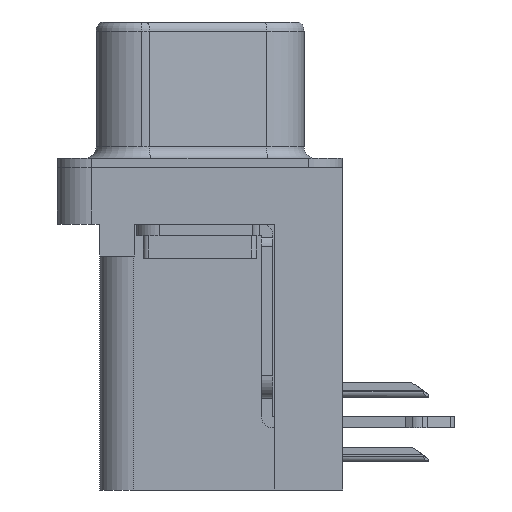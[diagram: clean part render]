
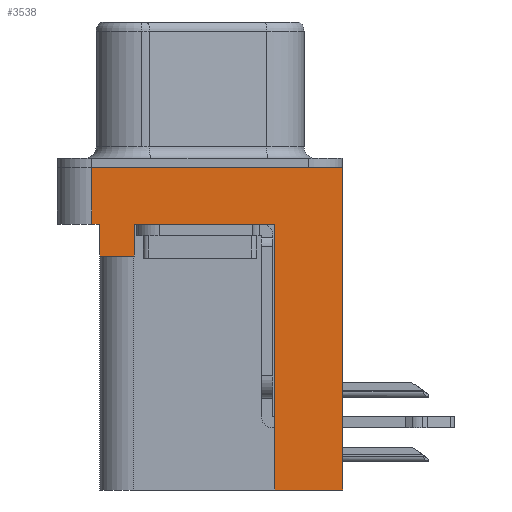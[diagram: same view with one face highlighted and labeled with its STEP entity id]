
A CAD part, left-side view. The second image highlights one B-rep face of the part: STEP entity #3538.
In plain terms, the highlighted planar face has unit normal (-1, 0, 0).
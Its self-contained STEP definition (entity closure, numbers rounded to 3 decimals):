
#238 = LINE ( 'NONE', #12211, #2899 ) ;
#440 = EDGE_CURVE ( 'NONE', #10118, #19211, #15057, .T. ) ;
#524 = CARTESIAN_POINT ( 'NONE',  ( -2.91, 4.775, -2.5 ) ) ;
#968 = DIRECTION ( 'NONE',  ( 0., -1., 0. ) ) ;
#1607 = CARTESIAN_POINT ( 'NONE',  ( -2.91, -3.295, -14.2 ) ) ;
#1790 = DIRECTION ( 'NONE',  ( 0., -1., 0. ) ) ;
#1872 = CARTESIAN_POINT ( 'NONE',  ( -2.91, -6.275, -14.2 ) ) ;
#1928 = LINE ( 'NONE', #10329, #10955 ) ;
#2899 = VECTOR ( 'NONE', #23032, 1000. ) ;
#2955 = ORIENTED_EDGE ( 'NONE', *, *, #18071, .F. ) ;
#3236 = FACE_OUTER_BOUND ( 'NONE', #4705, .T. ) ;
#3308 = VERTEX_POINT ( 'NONE', #25746 ) ;
#3538 = ADVANCED_FACE ( 'NONE', ( #3236 ), #11622, .T. ) ;
#3618 = CARTESIAN_POINT ( 'NONE',  ( -2.91, -3.295, -2.5 ) ) ;
#3626 = ORIENTED_EDGE ( 'NONE', *, *, #4228, .F. ) ;
#4175 = CARTESIAN_POINT ( 'NONE',  ( -2.91, 4.775, 0. ) ) ;
#4181 = ORIENTED_EDGE ( 'NONE', *, *, #12419, .T. ) ;
#4228 = EDGE_CURVE ( 'NONE', #21838, #14316, #9188, .T. ) ;
#4274 = EDGE_CURVE ( 'NONE', #10118, #15035, #8918, .T. ) ;
#4481 = VERTEX_POINT ( 'NONE', #1872 ) ;
#4495 = DIRECTION ( 'NONE',  ( 0., 0., 1. ) ) ;
#4705 = EDGE_LOOP ( 'NONE', ( #24730, #3626, #4181, #11059, #13642, #17425, #17779, #13672, #2955, #18287 ) ) ;
#5242 = VERTEX_POINT ( 'NONE', #1607 ) ;
#6165 = CARTESIAN_POINT ( 'NONE',  ( -2.91, -3.295, -14.2 ) ) ;
#6808 = LINE ( 'NONE', #7444, #15764 ) ;
#7237 = CARTESIAN_POINT ( 'NONE',  ( -2.91, 2.895, -2.5 ) ) ;
#7444 = CARTESIAN_POINT ( 'NONE',  ( -2.91, -6.275, -2.5 ) ) ;
#7488 = DIRECTION ( 'NONE',  ( 0., 0., 1. ) ) ;
#7683 = CARTESIAN_POINT ( 'NONE',  ( -2.91, 4.425, -3.9 ) ) ;
#7937 = EDGE_CURVE ( 'NONE', #5242, #17884, #26872, .T. ) ;
#8073 = DIRECTION ( 'NONE',  ( 0., 0., 1. ) ) ;
#8788 = VECTOR ( 'NONE', #19733, 1000. ) ;
#8872 = DIRECTION ( 'NONE',  ( 0., 0., 1. ) ) ;
#8918 = LINE ( 'NONE', #9320, #22481 ) ;
#9188 = LINE ( 'NONE', #524, #23735 ) ;
#9320 = CARTESIAN_POINT ( 'NONE',  ( -2.91, 4.425, -3.9 ) ) ;
#9418 = VECTOR ( 'NONE', #8073, 1000. ) ;
#10118 = VERTEX_POINT ( 'NONE', #10453 ) ;
#10329 = CARTESIAN_POINT ( 'NONE',  ( -2.91, -6.275, 0. ) ) ;
#10453 = CARTESIAN_POINT ( 'NONE',  ( -2.91, 2.895, -3.9 ) ) ;
#10955 = VECTOR ( 'NONE', #1790, 1000. ) ;
#11059 = ORIENTED_EDGE ( 'NONE', *, *, #20210, .F. ) ;
#11490 = CARTESIAN_POINT ( 'NONE',  ( -2.91, 4.775, -2.5 ) ) ;
#11622 = PLANE ( 'NONE',  #13136 ) ;
#11770 = EDGE_CURVE ( 'NONE', #4481, #17415, #6808, .T. ) ;
#11969 = EDGE_CURVE ( 'NONE', #14316, #17415, #1928, .T. ) ;
#12211 = CARTESIAN_POINT ( 'NONE',  ( -2.91, 4.425, -3.9 ) ) ;
#12419 = EDGE_CURVE ( 'NONE', #21838, #3308, #17669, .T. ) ;
#13136 = AXIS2_PLACEMENT_3D ( 'NONE', #26284, #17925, #7488 ) ;
#13312 = DIRECTION ( 'NONE',  ( 0., 1., 0. ) ) ;
#13642 = ORIENTED_EDGE ( 'NONE', *, *, #4274, .F. ) ;
#13672 = ORIENTED_EDGE ( 'NONE', *, *, #7937, .F. ) ;
#13702 = CARTESIAN_POINT ( 'NONE',  ( -2.91, -6.275, -2.5 ) ) ;
#14316 = VERTEX_POINT ( 'NONE', #4175 ) ;
#15035 = VERTEX_POINT ( 'NONE', #7683 ) ;
#15057 = LINE ( 'NONE', #26738, #26340 ) ;
#15143 = CARTESIAN_POINT ( 'NONE',  ( -2.91, -3.295, -14.2 ) ) ;
#15764 = VECTOR ( 'NONE', #4495, 1000. ) ;
#16016 = CARTESIAN_POINT ( 'NONE',  ( -2.91, -6.275, 0. ) ) ;
#17415 = VERTEX_POINT ( 'NONE', #16016 ) ;
#17425 = ORIENTED_EDGE ( 'NONE', *, *, #440, .T. ) ;
#17460 = LINE ( 'NONE', #25957, #19903 ) ;
#17468 = DIRECTION ( 'NONE',  ( 0., 1., 0. ) ) ;
#17669 = LINE ( 'NONE', #13702, #8788 ) ;
#17779 = ORIENTED_EDGE ( 'NONE', *, *, #22188, .T. ) ;
#17884 = VERTEX_POINT ( 'NONE', #3618 ) ;
#17925 = DIRECTION ( 'NONE',  ( -1., 0., 0. ) ) ;
#18071 = EDGE_CURVE ( 'NONE', #4481, #5242, #25965, .T. ) ;
#18287 = ORIENTED_EDGE ( 'NONE', *, *, #11770, .T. ) ;
#19211 = VERTEX_POINT ( 'NONE', #7237 ) ;
#19733 = DIRECTION ( 'NONE',  ( 0., -1., 0. ) ) ;
#19903 = VECTOR ( 'NONE', #968, 1000. ) ;
#20210 = EDGE_CURVE ( 'NONE', #15035, #3308, #238, .T. ) ;
#21629 = VECTOR ( 'NONE', #17468, 1000. ) ;
#21838 = VERTEX_POINT ( 'NONE', #11490 ) ;
#21932 = DIRECTION ( 'NONE',  ( 0., 0., 1. ) ) ;
#22188 = EDGE_CURVE ( 'NONE', #19211, #17884, #17460, .T. ) ;
#22481 = VECTOR ( 'NONE', #13312, 1000. ) ;
#23032 = DIRECTION ( 'NONE',  ( 0., 0., 1. ) ) ;
#23735 = VECTOR ( 'NONE', #21932, 1000. ) ;
#24730 = ORIENTED_EDGE ( 'NONE', *, *, #11969, .F. ) ;
#25746 = CARTESIAN_POINT ( 'NONE',  ( -2.91, 4.425, -2.5 ) ) ;
#25957 = CARTESIAN_POINT ( 'NONE',  ( -2.91, -6.275, -2.5 ) ) ;
#25965 = LINE ( 'NONE', #15143, #21629 ) ;
#26284 = CARTESIAN_POINT ( 'NONE',  ( -2.91, -6.275, -2.5 ) ) ;
#26340 = VECTOR ( 'NONE', #8872, 1000. ) ;
#26738 = CARTESIAN_POINT ( 'NONE',  ( -2.91, 2.895, -3.9 ) ) ;
#26872 = LINE ( 'NONE', #6165, #9418 ) ;
